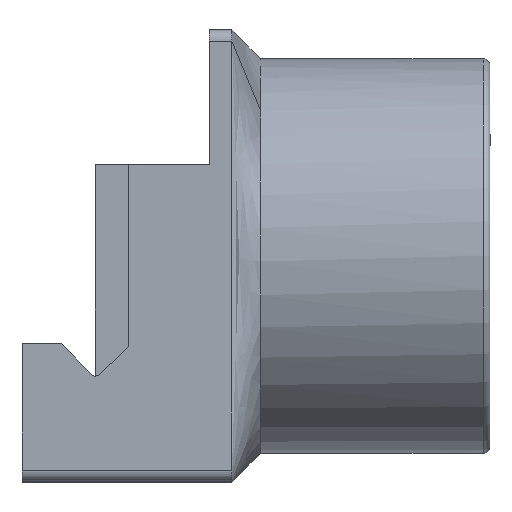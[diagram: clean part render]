
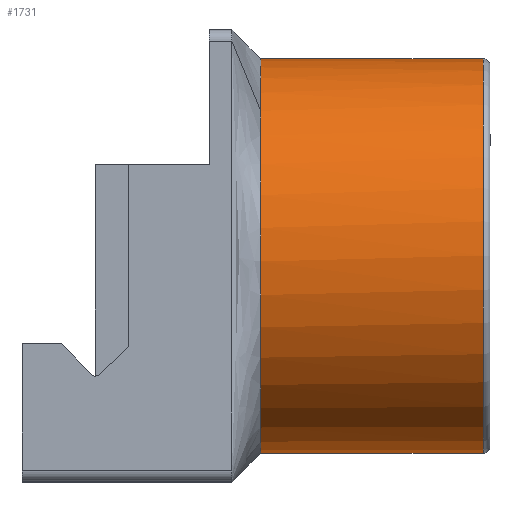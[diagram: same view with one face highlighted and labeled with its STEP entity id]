
A CAD part, top view. The second image highlights one B-rep face of the part: STEP entity #1731.
In plain terms, the highlighted cylindrical face has radius 17.462 mm (diameter 34.925 mm), a partial arc.
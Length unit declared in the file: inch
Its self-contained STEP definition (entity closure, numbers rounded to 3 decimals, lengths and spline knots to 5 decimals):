
#240 = CIRCLE ( 'NONE', #1749, 0.6875 ) ;
#446 = DIRECTION ( 'NONE',  ( -1., 0., 0. ) ) ;
#458 = VERTEX_POINT ( 'NONE', #3792 ) ;
#485 = VERTEX_POINT ( 'NONE', #2594 ) ;
#521 = CARTESIAN_POINT ( 'NONE',  ( 1.63228, 0.0999, 0.68898 ) ) ;
#607 = LINE ( 'NONE', #521, #4398 ) ;
#705 = DIRECTION ( 'NONE',  ( -1., 0., 0. ) ) ;
#784 = DIRECTION ( 'NONE',  ( 0., -1., 0. ) ) ;
#853 = CIRCLE ( 'NONE', #3957, 0.6875 ) ;
#1056 = ORIENTED_EDGE ( 'NONE', *, *, #2445, .F. ) ;
#1120 = ORIENTED_EDGE ( 'NONE', *, *, #2782, .T. ) ;
#1415 = CARTESIAN_POINT ( 'NONE',  ( 1.60847, 1.4749, 0.68898 ) ) ;
#1471 = EDGE_CURVE ( 'NONE', #1767, #2393, #240, .T. ) ;
#1724 = DIRECTION ( 'NONE',  ( 0., 1., 0. ) ) ;
#1731 = ADVANCED_FACE ( 'NONE', ( #4273 ), #5129, .T. ) ;
#1749 = AXIS2_PLACEMENT_3D ( 'NONE', #5380, #705, #784 ) ;
#1767 = VERTEX_POINT ( 'NONE', #3408 ) ;
#1795 = ORIENTED_EDGE ( 'NONE', *, *, #2208, .F. ) ;
#2012 = AXIS2_PLACEMENT_3D ( 'NONE', #4245, #446, #1724 ) ;
#2040 = CARTESIAN_POINT ( 'NONE',  ( 0.83228, 0.7874, 0.68898 ) ) ;
#2208 = EDGE_CURVE ( 'NONE', #458, #485, #607, .T. ) ;
#2331 = CARTESIAN_POINT ( 'NONE',  ( 1.63228, 1.4749, 0.68898 ) ) ;
#2393 = VERTEX_POINT ( 'NONE', #3386 ) ;
#2445 = EDGE_CURVE ( 'NONE', #485, #1767, #853, .T. ) ;
#2594 = CARTESIAN_POINT ( 'NONE',  ( 0.83228, 0.09989, 0.68898 ) ) ;
#2717 = VECTOR ( 'NONE', #4017, 39.37008 ) ;
#2782 = EDGE_CURVE ( 'NONE', #458, #4034, #5454, .T. ) ;
#2933 = DIRECTION ( 'NONE',  ( 0., -1., 0. ) ) ;
#3272 = ORIENTED_EDGE ( 'NONE', *, *, #3388, .T. ) ;
#3340 = AXIS2_PLACEMENT_3D ( 'NONE', #4159, #3771, #2933 ) ;
#3386 = CARTESIAN_POINT ( 'NONE',  ( 0.83228, 1.47491, 0.68898 ) ) ;
#3388 = EDGE_CURVE ( 'NONE', #4034, #2393, #3489, .T. ) ;
#3408 = CARTESIAN_POINT ( 'NONE',  ( 0.83228, 1.29309, 1.15474 ) ) ;
#3489 = LINE ( 'NONE', #2331, #2717 ) ;
#3623 = DIRECTION ( 'NONE',  ( 0., -1., 0. ) ) ;
#3771 = DIRECTION ( 'NONE',  ( -1., 0., 0. ) ) ;
#3792 = CARTESIAN_POINT ( 'NONE',  ( 1.60847, 0.0999, 0.68898 ) ) ;
#3957 = AXIS2_PLACEMENT_3D ( 'NONE', #2040, #5054, #3623 ) ;
#4017 = DIRECTION ( 'NONE',  ( -1., 0., 0. ) ) ;
#4034 = VERTEX_POINT ( 'NONE', #1415 ) ;
#4159 = CARTESIAN_POINT ( 'NONE',  ( 1.60847, 0.7874, 0.68898 ) ) ;
#4245 = CARTESIAN_POINT ( 'NONE',  ( 1.63228, 0.7874, 0.68898 ) ) ;
#4273 = FACE_OUTER_BOUND ( 'NONE', #4775, .T. ) ;
#4398 = VECTOR ( 'NONE', #4821, 39.37008 ) ;
#4585 = ORIENTED_EDGE ( 'NONE', *, *, #1471, .F. ) ;
#4775 = EDGE_LOOP ( 'NONE', ( #1795, #1120, #3272, #4585, #1056 ) ) ;
#4821 = DIRECTION ( 'NONE',  ( -1., 0., 0. ) ) ;
#5054 = DIRECTION ( 'NONE',  ( -1., 0., 0. ) ) ;
#5129 = CYLINDRICAL_SURFACE ( 'NONE', #2012, 0.6875 ) ;
#5380 = CARTESIAN_POINT ( 'NONE',  ( 0.83228, 0.7874, 0.68898 ) ) ;
#5454 = CIRCLE ( 'NONE', #3340, 0.6875 ) ;
